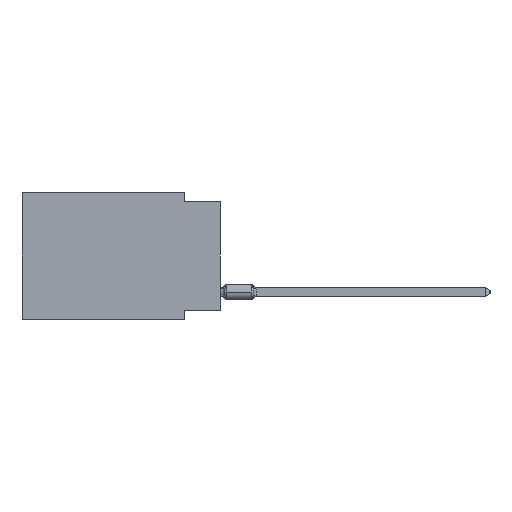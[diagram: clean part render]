
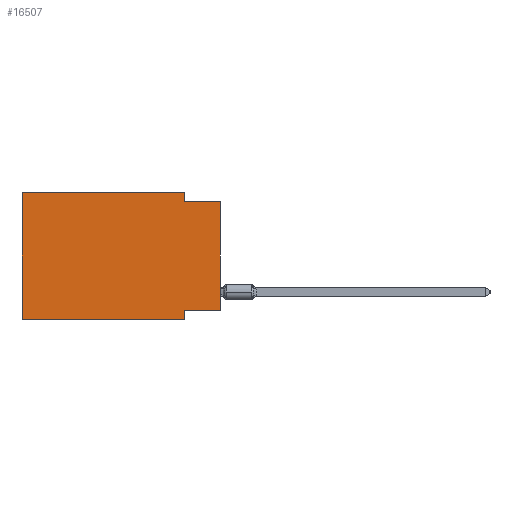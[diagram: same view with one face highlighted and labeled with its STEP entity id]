
A CAD part, left-side view. The second image highlights one B-rep face of the part: STEP entity #16507.
In plain terms, the highlighted planar face has unit normal (-1, 0, 0).
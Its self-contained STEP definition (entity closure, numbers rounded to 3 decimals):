
#53 = DIRECTION ( 'NONE',  ( 0., 0., 1. ) ) ;
#210 = ORIENTED_EDGE ( 'NONE', *, *, #28601, .T. ) ;
#1470 = VERTEX_POINT ( 'NONE', #40161 ) ;
#3083 = CARTESIAN_POINT ( 'NONE',  ( 0., 2.54, 0. ) ) ;
#4391 = EDGE_CURVE ( 'NONE', #51755, #30212, #37007, .T. ) ;
#5590 = VERTEX_POINT ( 'NONE', #50269 ) ;
#6615 = DIRECTION ( 'NONE',  ( 0., -1., 0. ) ) ;
#7834 = LINE ( 'NONE', #12958, #43529 ) ;
#8678 = CARTESIAN_POINT ( 'NONE',  ( 0., 2.54, -8.255 ) ) ;
#9645 = VECTOR ( 'NONE', #6615, 1000. ) ;
#10469 = VERTEX_POINT ( 'NONE', #19292 ) ;
#10719 = LINE ( 'NONE', #45706, #26274 ) ;
#12458 = LINE ( 'NONE', #12729, #21016 ) ;
#12520 = CARTESIAN_POINT ( 'NONE',  ( 0., 13.97, 0. ) ) ;
#12729 = CARTESIAN_POINT ( 'NONE',  ( 0., 2.54, 0. ) ) ;
#12917 = CARTESIAN_POINT ( 'NONE',  ( 0., 2.54, -8.89 ) ) ;
#12958 = CARTESIAN_POINT ( 'NONE',  ( 0., 13.97, 0. ) ) ;
#13769 = LINE ( 'NONE', #39317, #55681 ) ;
#14534 = VERTEX_POINT ( 'NONE', #3083 ) ;
#15627 = DIRECTION ( 'NONE',  ( 0., -1., 0. ) ) ;
#16507 = ADVANCED_FACE ( 'NONE', ( #34329 ), #34596, .F. ) ;
#17526 = CARTESIAN_POINT ( 'NONE',  ( 0., 13.97, 0. ) ) ;
#18418 = ORIENTED_EDGE ( 'NONE', *, *, #4391, .F. ) ;
#18478 = EDGE_CURVE ( 'NONE', #5590, #51079, #13769, .T. ) ;
#18663 = CARTESIAN_POINT ( 'NONE',  ( 0., 0., -0.635 ) ) ;
#19292 = CARTESIAN_POINT ( 'NONE',  ( 0., 2.54, -8.89 ) ) ;
#19680 = CARTESIAN_POINT ( 'NONE',  ( 0., 0., -0.635 ) ) ;
#19925 = EDGE_CURVE ( 'NONE', #51079, #10469, #30130, .T. ) ;
#20888 = ORIENTED_EDGE ( 'NONE', *, *, #22710, .T. ) ;
#21016 = VECTOR ( 'NONE', #47449, 1000. ) ;
#22342 = CARTESIAN_POINT ( 'NONE',  ( 0., 2.54, -0.635 ) ) ;
#22710 = EDGE_CURVE ( 'NONE', #5590, #30212, #50261, .T. ) ;
#26274 = VECTOR ( 'NONE', #33092, 1000. ) ;
#26521 = EDGE_CURVE ( 'NONE', #47667, #1470, #7834, .T. ) ;
#28601 = EDGE_CURVE ( 'NONE', #47667, #10469, #10719, .T. ) ;
#29564 = DIRECTION ( 'NONE',  ( 0., 0., -1. ) ) ;
#30008 = DIRECTION ( 'NONE',  ( 1., 0., 0. ) ) ;
#30044 = ORIENTED_EDGE ( 'NONE', *, *, #26521, .F. ) ;
#30130 = LINE ( 'NONE', #12917, #39226 ) ;
#30212 = VERTEX_POINT ( 'NONE', #19680 ) ;
#30421 = VECTOR ( 'NONE', #54007, 1000. ) ;
#32505 = ORIENTED_EDGE ( 'NONE', *, *, #35633, .F. ) ;
#33092 = DIRECTION ( 'NONE',  ( 0., -1., 0. ) ) ;
#33761 = CARTESIAN_POINT ( 'NONE',  ( 0., 13.97, -8.89 ) ) ;
#34329 = FACE_OUTER_BOUND ( 'NONE', #53912, .T. ) ;
#34596 = PLANE ( 'NONE',  #56380 ) ;
#35633 = EDGE_CURVE ( 'NONE', #1470, #14534, #54946, .T. ) ;
#36487 = CARTESIAN_POINT ( 'NONE',  ( 0., 0., 0. ) ) ;
#37007 = LINE ( 'NONE', #18663, #9645 ) ;
#38533 = EDGE_CURVE ( 'NONE', #14534, #51755, #12458, .T. ) ;
#38910 = DIRECTION ( 'NONE',  ( 0., 0., -1. ) ) ;
#39226 = VECTOR ( 'NONE', #29564, 1000. ) ;
#39317 = CARTESIAN_POINT ( 'NONE',  ( 0., 0., -8.255 ) ) ;
#40161 = CARTESIAN_POINT ( 'NONE',  ( 0., 13.97, 0. ) ) ;
#41493 = ORIENTED_EDGE ( 'NONE', *, *, #18478, .F. ) ;
#43529 = VECTOR ( 'NONE', #53, 1000. ) ;
#45706 = CARTESIAN_POINT ( 'NONE',  ( 0., 13.97, -8.89 ) ) ;
#47449 = DIRECTION ( 'NONE',  ( 0., 0., -1. ) ) ;
#47667 = VERTEX_POINT ( 'NONE', #33761 ) ;
#47938 = DIRECTION ( 'NONE',  ( 0., 1., 0. ) ) ;
#48112 = VECTOR ( 'NONE', #15627, 1000. ) ;
#50261 = LINE ( 'NONE', #36487, #30421 ) ;
#50269 = CARTESIAN_POINT ( 'NONE',  ( 0., 0., -8.255 ) ) ;
#51079 = VERTEX_POINT ( 'NONE', #8678 ) ;
#51755 = VERTEX_POINT ( 'NONE', #22342 ) ;
#53912 = EDGE_LOOP ( 'NONE', ( #20888, #18418, #55809, #32505, #30044, #210, #55996, #41493 ) ) ;
#54007 = DIRECTION ( 'NONE',  ( 0., 0., 1. ) ) ;
#54946 = LINE ( 'NONE', #17526, #48112 ) ;
#55681 = VECTOR ( 'NONE', #47938, 1000. ) ;
#55809 = ORIENTED_EDGE ( 'NONE', *, *, #38533, .F. ) ;
#55996 = ORIENTED_EDGE ( 'NONE', *, *, #19925, .F. ) ;
#56380 = AXIS2_PLACEMENT_3D ( 'NONE', #12520, #30008, #38910 ) ;
